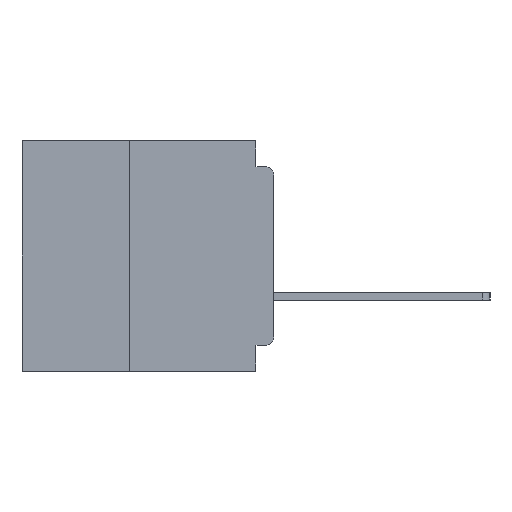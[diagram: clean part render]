
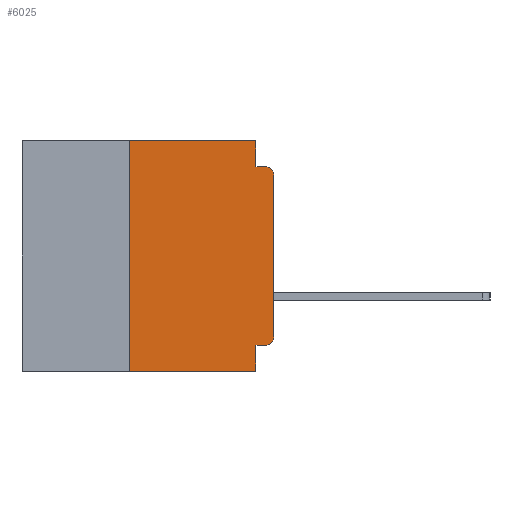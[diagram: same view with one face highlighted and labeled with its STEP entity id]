
A CAD part, left-side view. The second image highlights one B-rep face of the part: STEP entity #6025.
In plain terms, the highlighted planar face has unit normal (-1, 0, 0).
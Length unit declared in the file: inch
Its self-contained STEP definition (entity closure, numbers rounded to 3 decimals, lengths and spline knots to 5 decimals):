
#104 = CARTESIAN_POINT ( 'NONE',  ( 0., 0.031, -0.4 ) ) ;
#146 = VERTEX_POINT ( 'NONE', #44603 ) ;
#391 = CARTESIAN_POINT ( 'NONE',  ( 0., 0.031, 0. ) ) ;
#427 = CARTESIAN_POINT ( 'NONE',  ( 0., 0.031, -0.4 ) ) ;
#502 = ORIENTED_EDGE ( 'NONE', *, *, #26278, .F. ) ;
#1640 = DIRECTION ( 'NONE',  ( 0., 0., -1. ) ) ;
#1668 = EDGE_LOOP ( 'NONE', ( #20309, #42000, #33065, #502, #46520, #39950, #16749, #4259, #25535, #12397 ) ) ;
#2002 = CARTESIAN_POINT ( 'NONE',  ( 0., 0., -0.045 ) ) ;
#3284 = CARTESIAN_POINT ( 'NONE',  ( 0., 0.015, -0.34 ) ) ;
#3449 = CARTESIAN_POINT ( 'NONE',  ( 0., 0.25, 0. ) ) ;
#4259 = ORIENTED_EDGE ( 'NONE', *, *, #16310, .F. ) ;
#5729 = CARTESIAN_POINT ( 'NONE',  ( 0., 0.015, -0.355 ) ) ;
#6025 = ADVANCED_FACE ( 'NONE', ( #15649 ), #16869, .F. ) ;
#6289 = EDGE_CURVE ( 'NONE', #14212, #37781, #42285, .T. ) ;
#6963 = DIRECTION ( 'NONE',  ( 0., -1., 0. ) ) ;
#7134 = DIRECTION ( 'NONE',  ( 0., 0., -1. ) ) ;
#8527 = AXIS2_PLACEMENT_3D ( 'NONE', #35144, #12924, #38925 ) ;
#8799 = VERTEX_POINT ( 'NONE', #16102 ) ;
#9653 = VERTEX_POINT ( 'NONE', #40175 ) ;
#11747 = EDGE_CURVE ( 'NONE', #8799, #9653, #17578, .T. ) ;
#11785 = DIRECTION ( 'NONE',  ( 0., 1., 0. ) ) ;
#11798 = LINE ( 'NONE', #30562, #40321 ) ;
#12397 = ORIENTED_EDGE ( 'NONE', *, *, #18011, .T. ) ;
#12495 = EDGE_CURVE ( 'NONE', #26248, #9653, #42447, .T. ) ;
#12666 = CARTESIAN_POINT ( 'NONE',  ( 0., 0.25, -0.4 ) ) ;
#12924 = DIRECTION ( 'NONE',  ( -1., 0., 0. ) ) ;
#14212 = VERTEX_POINT ( 'NONE', #43599 ) ;
#14455 = CARTESIAN_POINT ( 'NONE',  ( 0., 0., -0.34 ) ) ;
#15215 = LINE ( 'NONE', #39755, #23970 ) ;
#15649 = FACE_OUTER_BOUND ( 'NONE', #1668, .T. ) ;
#15860 = LINE ( 'NONE', #41569, #24611 ) ;
#16102 = CARTESIAN_POINT ( 'NONE',  ( 0., 0., -0.06 ) ) ;
#16310 = EDGE_CURVE ( 'NONE', #146, #37781, #24718, .T. ) ;
#16449 = CIRCLE ( 'NONE', #16766, 0.015 ) ;
#16749 = ORIENTED_EDGE ( 'NONE', *, *, #6289, .T. ) ;
#16766 = AXIS2_PLACEMENT_3D ( 'NONE', #3284, #29569, #7134 ) ;
#16869 = PLANE ( 'NONE',  #35983 ) ;
#17460 = DIRECTION ( 'NONE',  ( 0., 0., 1. ) ) ;
#17578 = CIRCLE ( 'NONE', #8527, 0.015 ) ;
#18011 = EDGE_CURVE ( 'NONE', #20443, #22815, #16449, .T. ) ;
#18510 = EDGE_CURVE ( 'NONE', #22815, #8799, #15215, .T. ) ;
#20309 = ORIENTED_EDGE ( 'NONE', *, *, #18510, .T. ) ;
#20443 = VERTEX_POINT ( 'NONE', #5729 ) ;
#20616 = CARTESIAN_POINT ( 'NONE',  ( 0., 0.437, 0. ) ) ;
#21302 = LINE ( 'NONE', #12666, #29869 ) ;
#22669 = VECTOR ( 'NONE', #29567, 39.37008 ) ;
#22815 = VERTEX_POINT ( 'NONE', #14455 ) ;
#23335 = DIRECTION ( 'NONE',  ( 0., 0., -1. ) ) ;
#23970 = VECTOR ( 'NONE', #17460, 39.37008 ) ;
#24322 = DIRECTION ( 'NONE',  ( 1., 0., 0. ) ) ;
#24468 = VECTOR ( 'NONE', #6963, 39.37008 ) ;
#24611 = VECTOR ( 'NONE', #11785, 39.37008 ) ;
#24718 = LINE ( 'NONE', #427, #34432 ) ;
#25535 = ORIENTED_EDGE ( 'NONE', *, *, #36522, .F. ) ;
#25911 = CARTESIAN_POINT ( 'NONE',  ( 0., 0.437, -0.4 ) ) ;
#26248 = VERTEX_POINT ( 'NONE', #41616 ) ;
#26278 = EDGE_CURVE ( 'NONE', #46250, #26248, #11798, .T. ) ;
#28431 = VERTEX_POINT ( 'NONE', #3449 ) ;
#29567 = DIRECTION ( 'NONE',  ( 0., -1., 0. ) ) ;
#29569 = DIRECTION ( 'NONE',  ( -1., 0., 0. ) ) ;
#29869 = VECTOR ( 'NONE', #42426, 39.37008 ) ;
#30557 = DIRECTION ( 'NONE',  ( 0., 0., -1. ) ) ;
#30562 = CARTESIAN_POINT ( 'NONE',  ( 0., 0.031, 0. ) ) ;
#32958 = CARTESIAN_POINT ( 'NONE',  ( 0., 0.437, 0. ) ) ;
#33065 = ORIENTED_EDGE ( 'NONE', *, *, #12495, .F. ) ;
#34198 = LINE ( 'NONE', #32958, #24468 ) ;
#34432 = VECTOR ( 'NONE', #30557, 39.37008 ) ;
#35144 = CARTESIAN_POINT ( 'NONE',  ( 0., 0.015, -0.06 ) ) ;
#35983 = AXIS2_PLACEMENT_3D ( 'NONE', #20616, #24322, #1640 ) ;
#36522 = EDGE_CURVE ( 'NONE', #20443, #146, #15860, .T. ) ;
#37781 = VERTEX_POINT ( 'NONE', #104 ) ;
#38925 = DIRECTION ( 'NONE',  ( 0., 0., -1. ) ) ;
#39513 = DIRECTION ( 'NONE',  ( 0., -1., 0. ) ) ;
#39755 = CARTESIAN_POINT ( 'NONE',  ( 0., 0., 0. ) ) ;
#39950 = ORIENTED_EDGE ( 'NONE', *, *, #47503, .F. ) ;
#40175 = CARTESIAN_POINT ( 'NONE',  ( 0., 0.015, -0.045 ) ) ;
#40321 = VECTOR ( 'NONE', #23335, 39.37008 ) ;
#41313 = VECTOR ( 'NONE', #39513, 39.37008 ) ;
#41569 = CARTESIAN_POINT ( 'NONE',  ( 0., 0., -0.355 ) ) ;
#41616 = CARTESIAN_POINT ( 'NONE',  ( 0., 0.031, -0.045 ) ) ;
#42000 = ORIENTED_EDGE ( 'NONE', *, *, #11747, .T. ) ;
#42285 = LINE ( 'NONE', #25911, #22669 ) ;
#42426 = DIRECTION ( 'NONE',  ( 0., 0., 1. ) ) ;
#42447 = LINE ( 'NONE', #2002, #41313 ) ;
#43599 = CARTESIAN_POINT ( 'NONE',  ( 0., 0.25, -0.4 ) ) ;
#44157 = EDGE_CURVE ( 'NONE', #28431, #46250, #34198, .T. ) ;
#44603 = CARTESIAN_POINT ( 'NONE',  ( 0., 0.031, -0.355 ) ) ;
#46250 = VERTEX_POINT ( 'NONE', #391 ) ;
#46520 = ORIENTED_EDGE ( 'NONE', *, *, #44157, .F. ) ;
#47503 = EDGE_CURVE ( 'NONE', #14212, #28431, #21302, .T. ) ;
